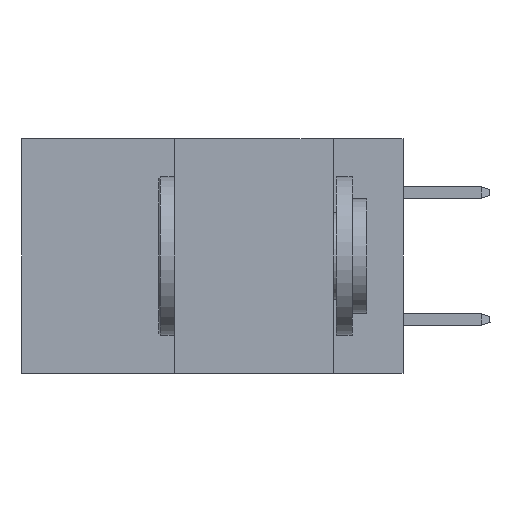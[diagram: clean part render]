
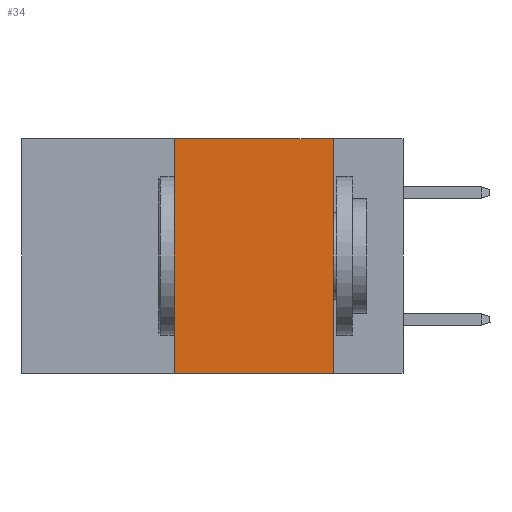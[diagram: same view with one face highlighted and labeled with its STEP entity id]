
A CAD part, left-side view. The second image highlights one B-rep face of the part: STEP entity #34.
In plain terms, the highlighted planar face has unit normal (-1, 0, 0).
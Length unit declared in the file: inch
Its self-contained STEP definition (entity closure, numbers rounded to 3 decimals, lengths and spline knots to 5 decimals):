
#34 = ADVANCED_FACE ( 'NONE', ( #16870 ), #17105, .F. ) ;
#118 = CARTESIAN_POINT ( 'NONE',  ( 0., 0.36, -0.37 ) ) ;
#632 = DIRECTION ( 'NONE',  ( 1., 0., 0. ) ) ;
#1146 = LINE ( 'NONE', #4932, #21273 ) ;
#2068 = VERTEX_POINT ( 'NONE', #118 ) ;
#2923 = VECTOR ( 'NONE', #14438, 39.37008 ) ;
#3001 = AXIS2_PLACEMENT_3D ( 'NONE', #8207, #632, #6433 ) ;
#3067 = VECTOR ( 'NONE', #19918, 39.37008 ) ;
#3358 = EDGE_CURVE ( 'NONE', #2068, #21135, #5451, .T. ) ;
#4932 = CARTESIAN_POINT ( 'NONE',  ( 0., 0.6, -0.37 ) ) ;
#5008 = EDGE_CURVE ( 'NONE', #2068, #13375, #1146, .T. ) ;
#5053 = DIRECTION ( 'NONE',  ( 0., -1., 0. ) ) ;
#5162 = CARTESIAN_POINT ( 'NONE',  ( 0., 0.6, 0. ) ) ;
#5451 = LINE ( 'NONE', #12660, #3067 ) ;
#6288 = EDGE_CURVE ( 'NONE', #21135, #10873, #20944, .T. ) ;
#6433 = DIRECTION ( 'NONE',  ( 0., 0., -1. ) ) ;
#7206 = CARTESIAN_POINT ( 'NONE',  ( 0., 0.11, 0. ) ) ;
#8135 = CARTESIAN_POINT ( 'NONE',  ( 0., 0.11, 0. ) ) ;
#8207 = CARTESIAN_POINT ( 'NONE',  ( 0., 0.6, 0. ) ) ;
#10298 = ORIENTED_EDGE ( 'NONE', *, *, #5008, .T. ) ;
#10873 = VERTEX_POINT ( 'NONE', #8135 ) ;
#11006 = ORIENTED_EDGE ( 'NONE', *, *, #3358, .F. ) ;
#11096 = LINE ( 'NONE', #7206, #2923 ) ;
#11766 = ORIENTED_EDGE ( 'NONE', *, *, #13068, .F. ) ;
#12660 = CARTESIAN_POINT ( 'NONE',  ( 0., 0.36, 0. ) ) ;
#13068 = EDGE_CURVE ( 'NONE', #10873, #13375, #11096, .T. ) ;
#13375 = VERTEX_POINT ( 'NONE', #19522 ) ;
#14101 = EDGE_LOOP ( 'NONE', ( #11766, #22077, #11006, #10298 ) ) ;
#14438 = DIRECTION ( 'NONE',  ( 0., 0., -1. ) ) ;
#15602 = DIRECTION ( 'NONE',  ( 0., -1., 0. ) ) ;
#16870 = FACE_OUTER_BOUND ( 'NONE', #14101, .T. ) ;
#17105 = PLANE ( 'NONE',  #3001 ) ;
#19522 = CARTESIAN_POINT ( 'NONE',  ( 0., 0.11, -0.37 ) ) ;
#19918 = DIRECTION ( 'NONE',  ( 0., 0., 1. ) ) ;
#20944 = LINE ( 'NONE', #5162, #22834 ) ;
#21135 = VERTEX_POINT ( 'NONE', #22190 ) ;
#21273 = VECTOR ( 'NONE', #15602, 39.37008 ) ;
#22077 = ORIENTED_EDGE ( 'NONE', *, *, #6288, .F. ) ;
#22190 = CARTESIAN_POINT ( 'NONE',  ( 0., 0.36, 0. ) ) ;
#22834 = VECTOR ( 'NONE', #5053, 39.37008 ) ;
